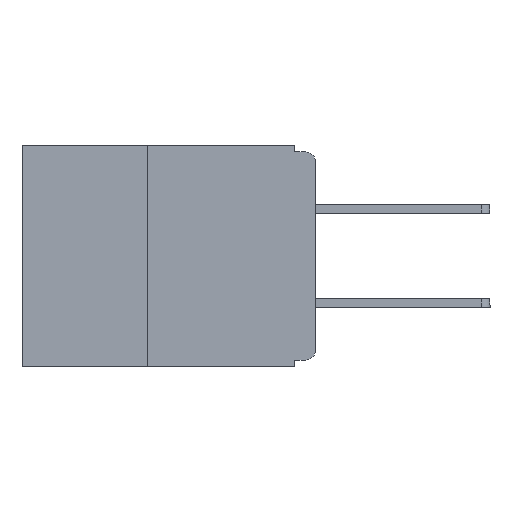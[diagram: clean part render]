
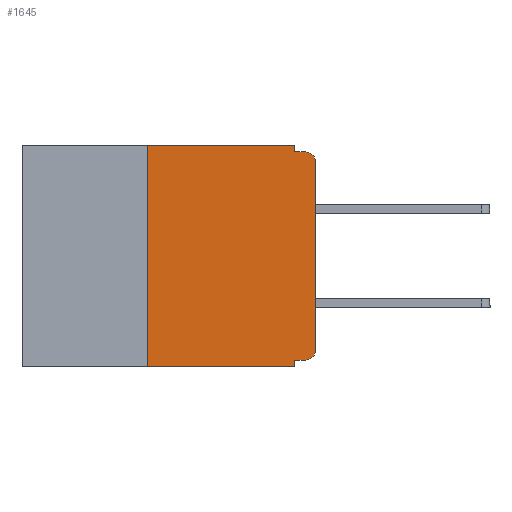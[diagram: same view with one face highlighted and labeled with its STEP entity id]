
A CAD part, left-side view. The second image highlights one B-rep face of the part: STEP entity #1645.
In plain terms, the highlighted planar face has unit normal (-1, 0, 0).
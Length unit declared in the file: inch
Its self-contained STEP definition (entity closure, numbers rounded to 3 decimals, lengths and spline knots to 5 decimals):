
#364 = LINE ( 'NONE', #16513, #1128 ) ;
#723 = EDGE_CURVE ( 'NONE', #14190, #25370, #18697, .T. ) ;
#768 = ORIENTED_EDGE ( 'NONE', *, *, #13953, .T. ) ;
#864 = ORIENTED_EDGE ( 'NONE', *, *, #5575, .T. ) ;
#980 = ORIENTED_EDGE ( 'NONE', *, *, #28416, .F. ) ;
#1128 = VECTOR ( 'NONE', #18892, 39.37008 ) ;
#1360 = CARTESIAN_POINT ( 'NONE',  ( 0., 0.031, -0.33 ) ) ;
#1631 = ORIENTED_EDGE ( 'NONE', *, *, #18663, .F. ) ;
#1645 = ADVANCED_FACE ( 'NONE', ( #29119 ), #29925, .F. ) ;
#1710 = ORIENTED_EDGE ( 'NONE', *, *, #31413, .F. ) ;
#1970 = VERTEX_POINT ( 'NONE', #2346 ) ;
#1987 = ORIENTED_EDGE ( 'NONE', *, *, #6283, .F. ) ;
#2142 = ORIENTED_EDGE ( 'NONE', *, *, #723, .T. ) ;
#2326 = ORIENTED_EDGE ( 'NONE', *, *, #13534, .F. ) ;
#2346 = CARTESIAN_POINT ( 'NONE',  ( 0., 0., -0.305 ) ) ;
#2775 = DIRECTION ( 'NONE',  ( 0., -1., 0. ) ) ;
#2826 = ORIENTED_EDGE ( 'NONE', *, *, #3584, .F. ) ;
#2960 = VECTOR ( 'NONE', #5660, 39.37008 ) ;
#3228 = ORIENTED_EDGE ( 'NONE', *, *, #14037, .T. ) ;
#3398 = VERTEX_POINT ( 'NONE', #29448 ) ;
#3584 = EDGE_CURVE ( 'NONE', #10616, #24657, #24200, .T. ) ;
#4756 = CARTESIAN_POINT ( 'NONE',  ( 0., 0.031, -0.33 ) ) ;
#5474 = VERTEX_POINT ( 'NONE', #29820 ) ;
#5575 = EDGE_CURVE ( 'NONE', #5474, #23360, #16622, .T. ) ;
#5660 = DIRECTION ( 'NONE',  ( 0., -1., 0. ) ) ;
#6012 = VERTEX_POINT ( 'NONE', #22011 ) ;
#6283 = EDGE_CURVE ( 'NONE', #14190, #11579, #8946, .T. ) ;
#6389 = DIRECTION ( 'NONE',  ( 0., 0., -1. ) ) ;
#7822 = LINE ( 'NONE', #27035, #27097 ) ;
#8441 = CARTESIAN_POINT ( 'NONE',  ( 0., 0.437, -0.33 ) ) ;
#8946 = LINE ( 'NONE', #17536, #14626 ) ;
#8957 = AXIS2_PLACEMENT_3D ( 'NONE', #20226, #17237, #6389 ) ;
#10616 = VERTEX_POINT ( 'NONE', #28925 ) ;
#11526 = VECTOR ( 'NONE', #18084, 39.37008 ) ;
#11579 = VERTEX_POINT ( 'NONE', #20440 ) ;
#12255 = CARTESIAN_POINT ( 'NONE',  ( 0., 0.25, -0.33 ) ) ;
#13534 = EDGE_CURVE ( 'NONE', #24657, #25370, #14278, .T. ) ;
#13747 = CARTESIAN_POINT ( 'NONE',  ( 0., 0., 0. ) ) ;
#13953 = EDGE_CURVE ( 'NONE', #1970, #5474, #27061, .T. ) ;
#14037 = EDGE_CURVE ( 'NONE', #10616, #1970, #19172, .T. ) ;
#14067 = CARTESIAN_POINT ( 'NONE',  ( 0., 0.015, -0.305 ) ) ;
#14190 = VERTEX_POINT ( 'NONE', #12255 ) ;
#14278 = LINE ( 'NONE', #4756, #26334 ) ;
#14432 = AXIS2_PLACEMENT_3D ( 'NONE', #14067, #30856, #16549 ) ;
#14498 = LINE ( 'NONE', #20241, #2960 ) ;
#14626 = VECTOR ( 'NONE', #17631, 39.37008 ) ;
#15800 = VECTOR ( 'NONE', #30547, 39.37008 ) ;
#16513 = CARTESIAN_POINT ( 'NONE',  ( 0., 0.031, 0. ) ) ;
#16549 = DIRECTION ( 'NONE',  ( 0., 0., -1. ) ) ;
#16622 = CIRCLE ( 'NONE', #29617, 0.015 ) ;
#16973 = DIRECTION ( 'NONE',  ( 0., 0., -1. ) ) ;
#17237 = DIRECTION ( 'NONE',  ( 1., 0., 0. ) ) ;
#17536 = CARTESIAN_POINT ( 'NONE',  ( 0., 0.25, -0.33 ) ) ;
#17631 = DIRECTION ( 'NONE',  ( 0., 0., 1. ) ) ;
#18084 = DIRECTION ( 'NONE',  ( 0., -1., 0. ) ) ;
#18663 = EDGE_CURVE ( 'NONE', #6012, #3398, #364, .T. ) ;
#18697 = LINE ( 'NONE', #8441, #11526 ) ;
#18892 = DIRECTION ( 'NONE',  ( 0., 0., -1. ) ) ;
#19172 = CIRCLE ( 'NONE', #14432, 0.015 ) ;
#20226 = CARTESIAN_POINT ( 'NONE',  ( 0., 0.437, 0. ) ) ;
#20241 = CARTESIAN_POINT ( 'NONE',  ( 0., 0.437, 0. ) ) ;
#20440 = CARTESIAN_POINT ( 'NONE',  ( 0., 0.25, 0. ) ) ;
#20559 = CARTESIAN_POINT ( 'NONE',  ( 0., 0.031, -0.32 ) ) ;
#21401 = DIRECTION ( 'NONE',  ( 0., 1., 0. ) ) ;
#22011 = CARTESIAN_POINT ( 'NONE',  ( 0., 0.031, 0. ) ) ;
#22549 = EDGE_LOOP ( 'NONE', ( #768, #864, #980, #1631, #1710, #1987, #2142, #2326, #2826, #3228 ) ) ;
#23360 = VERTEX_POINT ( 'NONE', #24796 ) ;
#24200 = LINE ( 'NONE', #28483, #29810 ) ;
#24657 = VERTEX_POINT ( 'NONE', #20559 ) ;
#24796 = CARTESIAN_POINT ( 'NONE',  ( 0., 0.015, -0.01 ) ) ;
#25370 = VERTEX_POINT ( 'NONE', #1360 ) ;
#26334 = VECTOR ( 'NONE', #16973, 39.37008 ) ;
#27035 = CARTESIAN_POINT ( 'NONE',  ( 0., 0., -0.01 ) ) ;
#27061 = LINE ( 'NONE', #13747, #15800 ) ;
#27097 = VECTOR ( 'NONE', #2775, 39.37008 ) ;
#28122 = DIRECTION ( 'NONE',  ( 0., 0., -1. ) ) ;
#28220 = DIRECTION ( 'NONE',  ( -1., 0., 0. ) ) ;
#28256 = CARTESIAN_POINT ( 'NONE',  ( 0., 0.015, -0.025 ) ) ;
#28416 = EDGE_CURVE ( 'NONE', #3398, #23360, #7822, .T. ) ;
#28483 = CARTESIAN_POINT ( 'NONE',  ( 0., 0., -0.32 ) ) ;
#28925 = CARTESIAN_POINT ( 'NONE',  ( 0., 0.015, -0.32 ) ) ;
#29119 = FACE_OUTER_BOUND ( 'NONE', #22549, .T. ) ;
#29448 = CARTESIAN_POINT ( 'NONE',  ( 0., 0.031, -0.01 ) ) ;
#29617 = AXIS2_PLACEMENT_3D ( 'NONE', #28256, #28220, #28122 ) ;
#29810 = VECTOR ( 'NONE', #21401, 39.37008 ) ;
#29820 = CARTESIAN_POINT ( 'NONE',  ( 0., 0., -0.025 ) ) ;
#29925 = PLANE ( 'NONE',  #8957 ) ;
#30547 = DIRECTION ( 'NONE',  ( 0., 0., 1. ) ) ;
#30856 = DIRECTION ( 'NONE',  ( -1., 0., 0. ) ) ;
#31413 = EDGE_CURVE ( 'NONE', #11579, #6012, #14498, .T. ) ;
